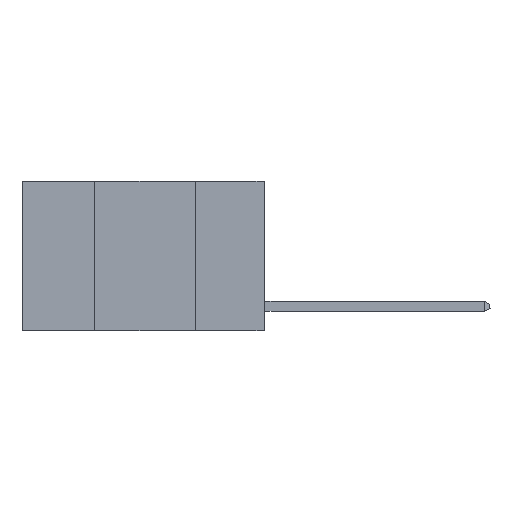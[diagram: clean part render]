
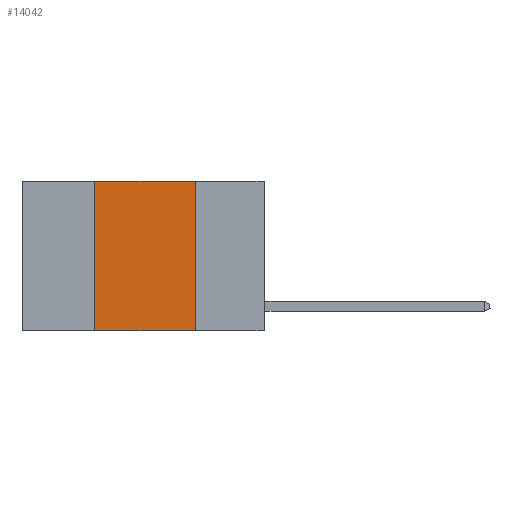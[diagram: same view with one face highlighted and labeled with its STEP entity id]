
A CAD part, left-side view. The second image highlights one B-rep face of the part: STEP entity #14042.
In plain terms, the highlighted planar face has unit normal (-1, 0, 0).
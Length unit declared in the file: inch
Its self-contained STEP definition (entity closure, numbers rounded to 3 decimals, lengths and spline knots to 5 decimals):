
#2427 = LINE ( 'NONE', #20169, #18408 ) ;
#2699 = VECTOR ( 'NONE', #19515, 39.37008 ) ;
#3362 = LINE ( 'NONE', #17443, #2699 ) ;
#3590 = PLANE ( 'NONE',  #9515 ) ;
#3684 = DIRECTION ( 'NONE',  ( 0., 0., -1. ) ) ;
#3781 = ORIENTED_EDGE ( 'NONE', *, *, #14839, .F. ) ;
#4303 = DIRECTION ( 'NONE',  ( 0., 0., -1. ) ) ;
#4810 = CARTESIAN_POINT ( 'NONE',  ( 0., 0.6, -0.37 ) ) ;
#5023 = EDGE_LOOP ( 'NONE', ( #3781, #26436, #16810, #9112 ) ) ;
#6592 = LINE ( 'NONE', #4810, #10836 ) ;
#7558 = FACE_OUTER_BOUND ( 'NONE', #5023, .T. ) ;
#8285 = VERTEX_POINT ( 'NONE', #23445 ) ;
#8573 = CARTESIAN_POINT ( 'NONE',  ( 0., 0.17, 0. ) ) ;
#9112 = ORIENTED_EDGE ( 'NONE', *, *, #20700, .T. ) ;
#9134 = VERTEX_POINT ( 'NONE', #22064 ) ;
#9515 = AXIS2_PLACEMENT_3D ( 'NONE', #20220, #16161, #3684 ) ;
#9842 = LINE ( 'NONE', #8573, #15293 ) ;
#9944 = DIRECTION ( 'NONE',  ( 0., 0., 1. ) ) ;
#10836 = VECTOR ( 'NONE', #21381, 39.37008 ) ;
#13799 = CARTESIAN_POINT ( 'NONE',  ( 0., 0.42, 0. ) ) ;
#14042 = ADVANCED_FACE ( 'NONE', ( #7558 ), #3590, .F. ) ;
#14839 = EDGE_CURVE ( 'NONE', #8285, #9134, #9842, .T. ) ;
#15293 = VECTOR ( 'NONE', #4303, 39.37008 ) ;
#16161 = DIRECTION ( 'NONE',  ( 1., 0., 0. ) ) ;
#16810 = ORIENTED_EDGE ( 'NONE', *, *, #26347, .F. ) ;
#17443 = CARTESIAN_POINT ( 'NONE',  ( 0., 0.6, 0. ) ) ;
#18265 = EDGE_CURVE ( 'NONE', #26291, #8285, #3362, .T. ) ;
#18408 = VECTOR ( 'NONE', #9944, 39.37008 ) ;
#19515 = DIRECTION ( 'NONE',  ( 0., -1., 0. ) ) ;
#20169 = CARTESIAN_POINT ( 'NONE',  ( 0., 0.42, 0. ) ) ;
#20220 = CARTESIAN_POINT ( 'NONE',  ( 0., 0.6, 0. ) ) ;
#20700 = EDGE_CURVE ( 'NONE', #21845, #9134, #6592, .T. ) ;
#21381 = DIRECTION ( 'NONE',  ( 0., -1., 0. ) ) ;
#21845 = VERTEX_POINT ( 'NONE', #22650 ) ;
#22064 = CARTESIAN_POINT ( 'NONE',  ( 0., 0.17, -0.37 ) ) ;
#22650 = CARTESIAN_POINT ( 'NONE',  ( 0., 0.42, -0.37 ) ) ;
#23445 = CARTESIAN_POINT ( 'NONE',  ( 0., 0.17, 0. ) ) ;
#26291 = VERTEX_POINT ( 'NONE', #13799 ) ;
#26347 = EDGE_CURVE ( 'NONE', #21845, #26291, #2427, .T. ) ;
#26436 = ORIENTED_EDGE ( 'NONE', *, *, #18265, .F. ) ;
